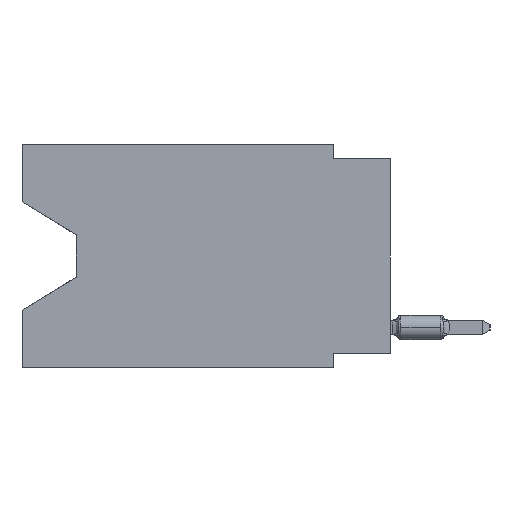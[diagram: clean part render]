
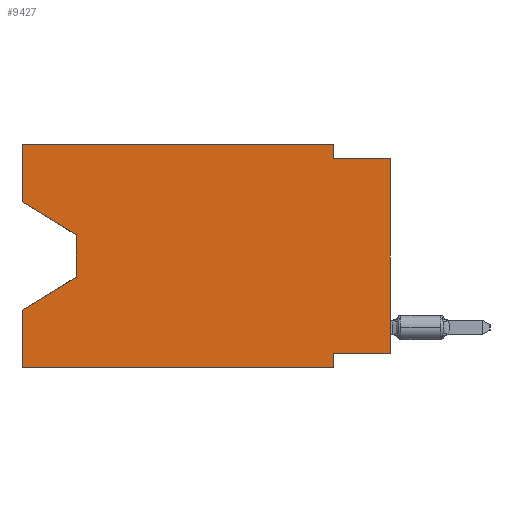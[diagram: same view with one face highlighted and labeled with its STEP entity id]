
A CAD part, left-side view. The second image highlights one B-rep face of the part: STEP entity #9427.
In plain terms, the highlighted planar face has unit normal (-1, 0, 0).
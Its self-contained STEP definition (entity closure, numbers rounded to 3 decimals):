
#346 = ORIENTED_EDGE ( 'NONE', *, *, #32700, .T. ) ;
#652 = LINE ( 'NONE', #25739, #51477 ) ;
#2744 = CARTESIAN_POINT ( 'NONE',  ( 0., 0., -0.635 ) ) ;
#2991 = ORIENTED_EDGE ( 'NONE', *, *, #10007, .T. ) ;
#3017 = DIRECTION ( 'NONE',  ( 0., 0., -1. ) ) ;
#3674 = ORIENTED_EDGE ( 'NONE', *, *, #53212, .F. ) ;
#3682 = LINE ( 'NONE', #56448, #13790 ) ;
#4272 = CARTESIAN_POINT ( 'NONE',  ( 0., 16.383, 0. ) ) ;
#4877 = DIRECTION ( 'NONE',  ( 1., 0., 0. ) ) ;
#6022 = LINE ( 'NONE', #42799, #54727 ) ;
#6342 = CARTESIAN_POINT ( 'NONE',  ( 0., 0., 0. ) ) ;
#7212 = VECTOR ( 'NONE', #15939, 1000. ) ;
#7220 = EDGE_CURVE ( 'NONE', #48280, #12263, #59928, .T. ) ;
#8027 = CARTESIAN_POINT ( 'NONE',  ( 0., 13.97, -5.893 ) ) ;
#8691 = CARTESIAN_POINT ( 'NONE',  ( 0., 16.383, 0. ) ) ;
#9271 = PLANE ( 'NONE',  #57574 ) ;
#9427 = ADVANCED_FACE ( 'NONE', ( #34060 ), #9271, .F. ) ;
#10007 = EDGE_CURVE ( 'NONE', #56594, #32549, #49360, .T. ) ;
#11802 = CARTESIAN_POINT ( 'NONE',  ( 0., 2.54, 0. ) ) ;
#12263 = VERTEX_POINT ( 'NONE', #32930 ) ;
#12746 = ORIENTED_EDGE ( 'NONE', *, *, #33960, .F. ) ;
#13790 = VECTOR ( 'NONE', #57672, 1000. ) ;
#15416 = CARTESIAN_POINT ( 'NONE',  ( 0., 2.54, 0. ) ) ;
#15547 = VECTOR ( 'NONE', #25477, 1000. ) ;
#15939 = DIRECTION ( 'NONE',  ( 0., 0., -1. ) ) ;
#16552 = LINE ( 'NONE', #35720, #36890 ) ;
#17210 = CARTESIAN_POINT ( 'NONE',  ( 0., 16.383, -9.906 ) ) ;
#18512 = ORIENTED_EDGE ( 'NONE', *, *, #29072, .F. ) ;
#18921 = DIRECTION ( 'NONE',  ( 0., 0.855, -0.519 ) ) ;
#18958 = CARTESIAN_POINT ( 'NONE',  ( 0., 0., -0.635 ) ) ;
#19489 = VERTEX_POINT ( 'NONE', #8027 ) ;
#19644 = LINE ( 'NONE', #54182, #50514 ) ;
#19795 = DIRECTION ( 'NONE',  ( 0., -1., 0. ) ) ;
#22904 = CARTESIAN_POINT ( 'NONE',  ( 0., 0., -9.271 ) ) ;
#23974 = CARTESIAN_POINT ( 'NONE',  ( 0., 16.383, -2.546 ) ) ;
#24479 = VERTEX_POINT ( 'NONE', #23974 ) ;
#24982 = EDGE_CURVE ( 'NONE', #24479, #37191, #19644, .T. ) ;
#25283 = DIRECTION ( 'NONE',  ( 0., 0., 1. ) ) ;
#25477 = DIRECTION ( 'NONE',  ( 0., 0., 1. ) ) ;
#25739 = CARTESIAN_POINT ( 'NONE',  ( 0., 16.383, 0. ) ) ;
#26592 = DIRECTION ( 'NONE',  ( 0., -0.855, -0.519 ) ) ;
#28469 = ORIENTED_EDGE ( 'NONE', *, *, #28631, .F. ) ;
#28631 = EDGE_CURVE ( 'NONE', #36176, #32549, #34012, .T. ) ;
#29072 = EDGE_CURVE ( 'NONE', #37191, #54558, #652, .T. ) ;
#30627 = LINE ( 'NONE', #34733, #62079 ) ;
#31811 = EDGE_CURVE ( 'NONE', #56594, #52775, #61866, .T. ) ;
#32019 = DIRECTION ( 'NONE',  ( 0., 1., 0. ) ) ;
#32322 = VECTOR ( 'NONE', #45779, 1000. ) ;
#32549 = VERTEX_POINT ( 'NONE', #2744 ) ;
#32629 = EDGE_CURVE ( 'NONE', #24479, #56625, #16552, .T. ) ;
#32700 = EDGE_CURVE ( 'NONE', #56625, #19489, #3682, .T. ) ;
#32930 = CARTESIAN_POINT ( 'NONE',  ( 0., 2.54, -9.906 ) ) ;
#33960 = EDGE_CURVE ( 'NONE', #48280, #43221, #30627, .T. ) ;
#34012 = LINE ( 'NONE', #18958, #55478 ) ;
#34060 = FACE_OUTER_BOUND ( 'NONE', #38030, .T. ) ;
#34590 = CARTESIAN_POINT ( 'NONE',  ( 0., 16.383, -7.36 ) ) ;
#34733 = CARTESIAN_POINT ( 'NONE',  ( 0., 16.383, 0. ) ) ;
#35720 = CARTESIAN_POINT ( 'NONE',  ( 0., 16.383, -2.546 ) ) ;
#36176 = VERTEX_POINT ( 'NONE', #46838 ) ;
#36890 = VECTOR ( 'NONE', #26592, 1000. ) ;
#37191 = VERTEX_POINT ( 'NONE', #8691 ) ;
#38030 = EDGE_LOOP ( 'NONE', ( #45148, #346, #59711, #12746, #48076, #3674, #55404, #2991, #28469, #43725, #18512, #46435 ) ) ;
#38123 = DIRECTION ( 'NONE',  ( 0., -1., 0. ) ) ;
#38431 = CARTESIAN_POINT ( 'NONE',  ( 0., 2.54, -9.271 ) ) ;
#38784 = DIRECTION ( 'NONE',  ( 0., 0., -1. ) ) ;
#41013 = LINE ( 'NONE', #11802, #55699 ) ;
#42799 = CARTESIAN_POINT ( 'NONE',  ( 0., 13.97, -5.893 ) ) ;
#43221 = VERTEX_POINT ( 'NONE', #34590 ) ;
#43725 = ORIENTED_EDGE ( 'NONE', *, *, #57361, .F. ) ;
#45148 = ORIENTED_EDGE ( 'NONE', *, *, #32629, .T. ) ;
#45779 = DIRECTION ( 'NONE',  ( 0., -1., 0. ) ) ;
#46435 = ORIENTED_EDGE ( 'NONE', *, *, #24982, .F. ) ;
#46838 = CARTESIAN_POINT ( 'NONE',  ( 0., 2.54, -0.635 ) ) ;
#48076 = ORIENTED_EDGE ( 'NONE', *, *, #7220, .T. ) ;
#48280 = VERTEX_POINT ( 'NONE', #61069 ) ;
#48615 = CARTESIAN_POINT ( 'NONE',  ( 0., 2.54, -9.906 ) ) ;
#48840 = VECTOR ( 'NONE', #32019, 1000. ) ;
#49360 = LINE ( 'NONE', #6342, #15547 ) ;
#49729 = CARTESIAN_POINT ( 'NONE',  ( 0., 13.97, -4.013 ) ) ;
#50514 = VECTOR ( 'NONE', #25283, 1000. ) ;
#51477 = VECTOR ( 'NONE', #19795, 1000. ) ;
#52775 = VERTEX_POINT ( 'NONE', #38431 ) ;
#53212 = EDGE_CURVE ( 'NONE', #52775, #12263, #58979, .T. ) ;
#54129 = CARTESIAN_POINT ( 'NONE',  ( 0., 0., -9.271 ) ) ;
#54182 = CARTESIAN_POINT ( 'NONE',  ( 0., 16.383, 0. ) ) ;
#54187 = DIRECTION ( 'NONE',  ( 0., 0., 1. ) ) ;
#54558 = VERTEX_POINT ( 'NONE', #15416 ) ;
#54727 = VECTOR ( 'NONE', #18921, 1000. ) ;
#55404 = ORIENTED_EDGE ( 'NONE', *, *, #31811, .F. ) ;
#55478 = VECTOR ( 'NONE', #38123, 1000. ) ;
#55699 = VECTOR ( 'NONE', #3017, 1000. ) ;
#56448 = CARTESIAN_POINT ( 'NONE',  ( 0., 13.97, -4.013 ) ) ;
#56594 = VERTEX_POINT ( 'NONE', #54129 ) ;
#56625 = VERTEX_POINT ( 'NONE', #49729 ) ;
#57361 = EDGE_CURVE ( 'NONE', #54558, #36176, #41013, .T. ) ;
#57574 = AXIS2_PLACEMENT_3D ( 'NONE', #4272, #4877, #38784 ) ;
#57672 = DIRECTION ( 'NONE',  ( 0., 0., -1. ) ) ;
#58154 = EDGE_CURVE ( 'NONE', #19489, #43221, #6022, .T. ) ;
#58979 = LINE ( 'NONE', #48615, #7212 ) ;
#59711 = ORIENTED_EDGE ( 'NONE', *, *, #58154, .T. ) ;
#59928 = LINE ( 'NONE', #17210, #32322 ) ;
#61069 = CARTESIAN_POINT ( 'NONE',  ( 0., 16.383, -9.906 ) ) ;
#61866 = LINE ( 'NONE', #22904, #48840 ) ;
#62079 = VECTOR ( 'NONE', #54187, 1000. ) ;
